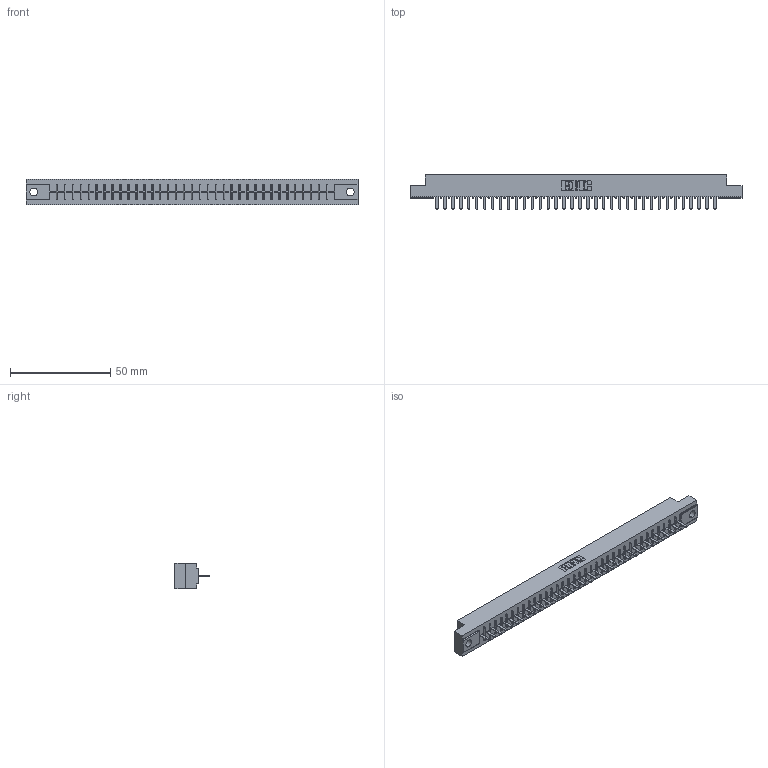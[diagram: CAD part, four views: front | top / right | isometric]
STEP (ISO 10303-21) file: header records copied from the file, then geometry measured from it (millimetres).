
FILE_DESCRIPTION (( 'STEP AP203' ), '1' );
FILE_NAME ('316-036-520-104.STEP', '2018-07-31T04:28:35', ( '' ), ( '' ), 'SwSTEP 2.0', 'SolidWorks 2016', '' );
FILE_SCHEMA (( 'CONFIG_CONTROL_DESIGN' ));
Length unit declared in the file: inch
Products named in the file (3): 316-036-520-104; 306 Part_.156 Dia; 306-290-001_120
Assembly tree (37 placements, depth 2):
  316-036-520-104
    306 Part_.156 Dia
    306-290-001_120  x36
Bounding box: 165.66 x 17.12 x 12.7 mm (x, y, z)
Volume: 18171.2 mm3; surface area: 18406.3 mm2
Topology: 37 solids, 37 shells, 2650 faces, 7444 edges, 4768 vertices
Faces by surface type: plane 1774, cylinder 732, sphere 144
Entity records: 34723 total; most frequent: CARTESIAN_POINT 5833, ORIENTED_EDGE 5780, DIRECTION 5744, EDGE_CURVE 2890, VECTOR 2266, LINE 2266, VERTEX_POINT 1828, AXIS2_PLACEMENT_3D 1739
